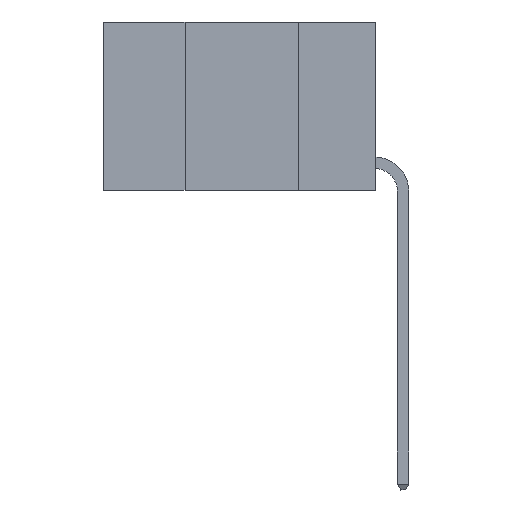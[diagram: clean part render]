
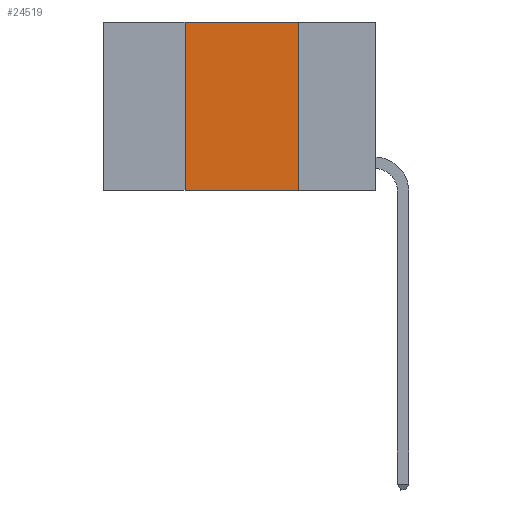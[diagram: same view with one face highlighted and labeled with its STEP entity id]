
A CAD part, left-side view. The second image highlights one B-rep face of the part: STEP entity #24519.
In plain terms, the highlighted planar face has unit normal (-1, 0, 0).
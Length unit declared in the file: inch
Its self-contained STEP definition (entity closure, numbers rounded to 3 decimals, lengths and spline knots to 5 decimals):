
#466 = VERTEX_POINT ( 'NONE', #8890 ) ;
#834 = DIRECTION ( 'NONE',  ( 0., -1., 0. ) ) ;
#1809 = CARTESIAN_POINT ( 'NONE',  ( 0., 0.6, 0. ) ) ;
#1960 = FACE_OUTER_BOUND ( 'NONE', #19223, .T. ) ;
#2199 = CARTESIAN_POINT ( 'NONE',  ( 0., 0.17, 0. ) ) ;
#2289 = ORIENTED_EDGE ( 'NONE', *, *, #19782, .F. ) ;
#2908 = LINE ( 'NONE', #18805, #20306 ) ;
#5549 = VECTOR ( 'NONE', #6376, 39.37008 ) ;
#6376 = DIRECTION ( 'NONE',  ( 0., 0., -1. ) ) ;
#7859 = VECTOR ( 'NONE', #834, 39.37008 ) ;
#8890 = CARTESIAN_POINT ( 'NONE',  ( 0., 0.17, -0.37 ) ) ;
#9002 = DIRECTION ( 'NONE',  ( 0., 0., 1. ) ) ;
#10964 = DIRECTION ( 'NONE',  ( 1., 0., 0. ) ) ;
#11103 = DIRECTION ( 'NONE',  ( 0., 0., -1. ) ) ;
#13770 = AXIS2_PLACEMENT_3D ( 'NONE', #1809, #10964, #11103 ) ;
#13952 = DIRECTION ( 'NONE',  ( 0., -1., 0. ) ) ;
#14894 = ORIENTED_EDGE ( 'NONE', *, *, #27581, .F. ) ;
#14971 = VERTEX_POINT ( 'NONE', #24262 ) ;
#15612 = CARTESIAN_POINT ( 'NONE',  ( 0., 0.42, 0. ) ) ;
#15867 = ORIENTED_EDGE ( 'NONE', *, *, #19331, .F. ) ;
#17061 = ORIENTED_EDGE ( 'NONE', *, *, #23795, .T. ) ;
#17780 = VECTOR ( 'NONE', #9002, 39.37008 ) ;
#18805 = CARTESIAN_POINT ( 'NONE',  ( 0., 0.6, -0.37 ) ) ;
#19223 = EDGE_LOOP ( 'NONE', ( #15867, #14894, #2289, #17061 ) ) ;
#19331 = EDGE_CURVE ( 'NONE', #19342, #466, #22682, .T. ) ;
#19342 = VERTEX_POINT ( 'NONE', #22536 ) ;
#19583 = CARTESIAN_POINT ( 'NONE',  ( 0., 0.42, -0.37 ) ) ;
#19782 = EDGE_CURVE ( 'NONE', #28956, #14971, #22066, .T. ) ;
#20306 = VECTOR ( 'NONE', #13952, 39.37008 ) ;
#21036 = CARTESIAN_POINT ( 'NONE',  ( 0., 0.6, 0. ) ) ;
#22066 = LINE ( 'NONE', #15612, #17780 ) ;
#22536 = CARTESIAN_POINT ( 'NONE',  ( 0., 0.17, 0. ) ) ;
#22682 = LINE ( 'NONE', #2199, #5549 ) ;
#23795 = EDGE_CURVE ( 'NONE', #28956, #466, #2908, .T. ) ;
#24262 = CARTESIAN_POINT ( 'NONE',  ( 0., 0.42, 0. ) ) ;
#24519 = ADVANCED_FACE ( 'NONE', ( #1960 ), #25074, .F. ) ;
#25074 = PLANE ( 'NONE',  #13770 ) ;
#25489 = LINE ( 'NONE', #21036, #7859 ) ;
#27581 = EDGE_CURVE ( 'NONE', #14971, #19342, #25489, .T. ) ;
#28956 = VERTEX_POINT ( 'NONE', #19583 ) ;
